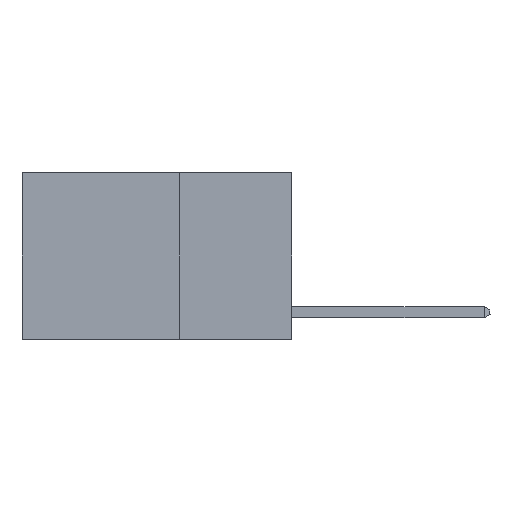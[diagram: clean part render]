
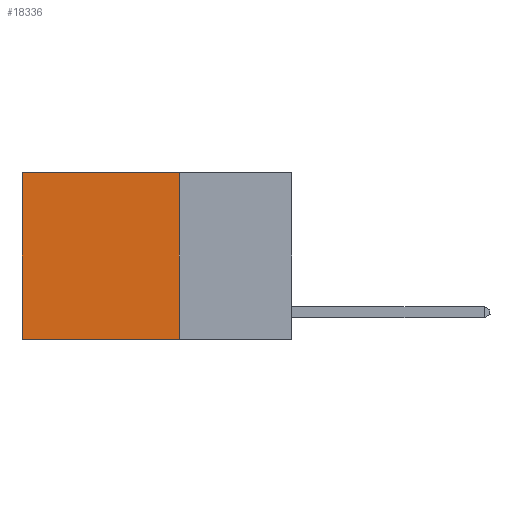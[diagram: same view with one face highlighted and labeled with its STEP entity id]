
A CAD part, left-side view. The second image highlights one B-rep face of the part: STEP entity #18336.
In plain terms, the highlighted planar face has unit normal (-1, 0, 0).
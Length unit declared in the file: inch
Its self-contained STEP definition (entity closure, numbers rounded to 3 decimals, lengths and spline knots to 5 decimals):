
#63 = EDGE_CURVE ( 'NONE', #6623, #15224, #13175, .T. ) ;
#863 = PLANE ( 'NONE',  #13026 ) ;
#2343 = ORIENTED_EDGE ( 'NONE', *, *, #8803, .T. ) ;
#2379 = DIRECTION ( 'NONE',  ( 1., 0., 0. ) ) ;
#2776 = CARTESIAN_POINT ( 'NONE',  ( 0.2625, 0.25, 0. ) ) ;
#3176 = DIRECTION ( 'NONE',  ( 0., 1., 0. ) ) ;
#3733 = VERTEX_POINT ( 'NONE', #18420 ) ;
#4085 = EDGE_LOOP ( 'NONE', ( #2343, #5978, #10590, #13134 ) ) ;
#4121 = EDGE_CURVE ( 'NONE', #17771, #6623, #16566, .T. ) ;
#4230 = CARTESIAN_POINT ( 'NONE',  ( 0.2625, 0.25, -0.37 ) ) ;
#5978 = ORIENTED_EDGE ( 'NONE', *, *, #63, .F. ) ;
#6148 = EDGE_CURVE ( 'NONE', #17771, #3733, #14893, .T. ) ;
#6623 = VERTEX_POINT ( 'NONE', #4230 ) ;
#8541 = VECTOR ( 'NONE', #13487, 39.37008 ) ;
#8733 = CARTESIAN_POINT ( 'NONE',  ( 0.2625, 0.25, 0. ) ) ;
#8803 = EDGE_CURVE ( 'NONE', #3733, #15224, #15800, .T. ) ;
#10190 = DIRECTION ( 'NONE',  ( 0., 1., 0. ) ) ;
#10539 = CARTESIAN_POINT ( 'NONE',  ( 0.2625, 0.6, 0. ) ) ;
#10590 = ORIENTED_EDGE ( 'NONE', *, *, #4121, .F. ) ;
#11029 = VECTOR ( 'NONE', #10190, 39.37008 ) ;
#11147 = CARTESIAN_POINT ( 'NONE',  ( 0.2625, 0.25, 0. ) ) ;
#11171 = CARTESIAN_POINT ( 'NONE',  ( 0.2625, 0.6, -0.37 ) ) ;
#11917 = CARTESIAN_POINT ( 'NONE',  ( 0.2625, 0.25, -0.37 ) ) ;
#12618 = DIRECTION ( 'NONE',  ( 0., 0., -1. ) ) ;
#13009 = DIRECTION ( 'NONE',  ( 0., 0., -1. ) ) ;
#13026 = AXIS2_PLACEMENT_3D ( 'NONE', #11147, #2379, #12618 ) ;
#13134 = ORIENTED_EDGE ( 'NONE', *, *, #6148, .T. ) ;
#13175 = LINE ( 'NONE', #11917, #16571 ) ;
#13487 = DIRECTION ( 'NONE',  ( 0., 0., -1. ) ) ;
#14176 = FACE_OUTER_BOUND ( 'NONE', #4085, .T. ) ;
#14893 = LINE ( 'NONE', #8733, #11029 ) ;
#15224 = VERTEX_POINT ( 'NONE', #11171 ) ;
#15800 = LINE ( 'NONE', #10539, #8541 ) ;
#16566 = LINE ( 'NONE', #2776, #18648 ) ;
#16571 = VECTOR ( 'NONE', #3176, 39.37008 ) ;
#17771 = VERTEX_POINT ( 'NONE', #18700 ) ;
#18336 = ADVANCED_FACE ( 'NONE', ( #14176 ), #863, .F. ) ;
#18420 = CARTESIAN_POINT ( 'NONE',  ( 0.2625, 0.6, 0. ) ) ;
#18648 = VECTOR ( 'NONE', #13009, 39.37008 ) ;
#18700 = CARTESIAN_POINT ( 'NONE',  ( 0.2625, 0.25, 0. ) ) ;
